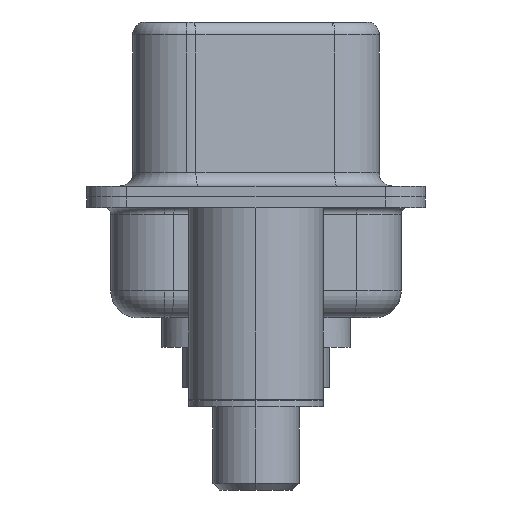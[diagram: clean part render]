
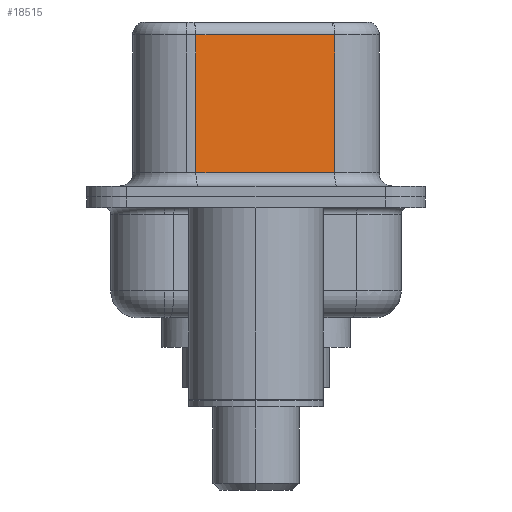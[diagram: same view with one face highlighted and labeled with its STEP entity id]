
A CAD part, left-side view. The second image highlights one B-rep face of the part: STEP entity #18515.
In plain terms, the highlighted planar face has unit normal (-0.985, -0.174, 0).
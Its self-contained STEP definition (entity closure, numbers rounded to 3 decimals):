
#870 = EDGE_CURVE ( 'NONE', #18856, #4158, #15404, .T. ) ;
#1180 = EDGE_CURVE ( 'NONE', #8654, #4158, #4343, .T. ) ;
#1417 = LINE ( 'NONE', #10471, #5296 ) ;
#1506 = VERTEX_POINT ( 'NONE', #18243 ) ;
#1547 = EDGE_CURVE ( 'NONE', #8654, #1506, #1417, .T. ) ;
#1825 = DIRECTION ( 'NONE',  ( 0., 0., -1. ) ) ;
#3019 = AXIS2_PLACEMENT_3D ( 'NONE', #18805, #7938, #9463 ) ;
#4158 = VERTEX_POINT ( 'NONE', #16319 ) ;
#4212 = VECTOR ( 'NONE', #1825, 1000. ) ;
#4343 = LINE ( 'NONE', #11924, #9010 ) ;
#5189 = EDGE_CURVE ( 'NONE', #1506, #18856, #18939, .T. ) ;
#5296 = VECTOR ( 'NONE', #10615, 1000. ) ;
#5903 = CARTESIAN_POINT ( 'NONE',  ( 4.58, -2.927, 0.9 ) ) ;
#6316 = VECTOR ( 'NONE', #19953, 1000. ) ;
#7938 = DIRECTION ( 'NONE',  ( 0.985, 0.174, 0. ) ) ;
#8260 = ORIENTED_EDGE ( 'NONE', *, *, #5189, .T. ) ;
#8654 = VERTEX_POINT ( 'NONE', #9938 ) ;
#9010 = VECTOR ( 'NONE', #13496, 1000. ) ;
#9463 = DIRECTION ( 'NONE',  ( -0.174, 0.985, 0. ) ) ;
#9585 = EDGE_LOOP ( 'NONE', ( #10140, #10734, #8260, #17590 ) ) ;
#9938 = CARTESIAN_POINT ( 'NONE',  ( 4.58, -2.927, 6.02 ) ) ;
#10058 = CARTESIAN_POINT ( 'NONE',  ( 3.67, 2.233, 0.9 ) ) ;
#10140 = ORIENTED_EDGE ( 'NONE', *, *, #1180, .F. ) ;
#10471 = CARTESIAN_POINT ( 'NONE',  ( 4.58, -2.927, 6.02 ) ) ;
#10615 = DIRECTION ( 'NONE',  ( -0.174, 0.985, 0. ) ) ;
#10734 = ORIENTED_EDGE ( 'NONE', *, *, #1547, .T. ) ;
#11924 = CARTESIAN_POINT ( 'NONE',  ( 4.58, -2.927, 6.52 ) ) ;
#13496 = DIRECTION ( 'NONE',  ( 0., 0., -1. ) ) ;
#14286 = CARTESIAN_POINT ( 'NONE',  ( 3.67, 2.233, 6.52 ) ) ;
#15404 = LINE ( 'NONE', #5903, #6316 ) ;
#16269 = FACE_OUTER_BOUND ( 'NONE', #9585, .T. ) ;
#16319 = CARTESIAN_POINT ( 'NONE',  ( 4.58, -2.927, 0.9 ) ) ;
#17590 = ORIENTED_EDGE ( 'NONE', *, *, #870, .T. ) ;
#18243 = CARTESIAN_POINT ( 'NONE',  ( 3.67, 2.233, 6.02 ) ) ;
#18465 = PLANE ( 'NONE',  #3019 ) ;
#18515 = ADVANCED_FACE ( 'NONE', ( #16269 ), #18465, .F. ) ;
#18805 = CARTESIAN_POINT ( 'NONE',  ( 4.58, -2.927, 6.52 ) ) ;
#18856 = VERTEX_POINT ( 'NONE', #10058 ) ;
#18939 = LINE ( 'NONE', #14286, #4212 ) ;
#19953 = DIRECTION ( 'NONE',  ( 0.174, -0.985, 0. ) ) ;
